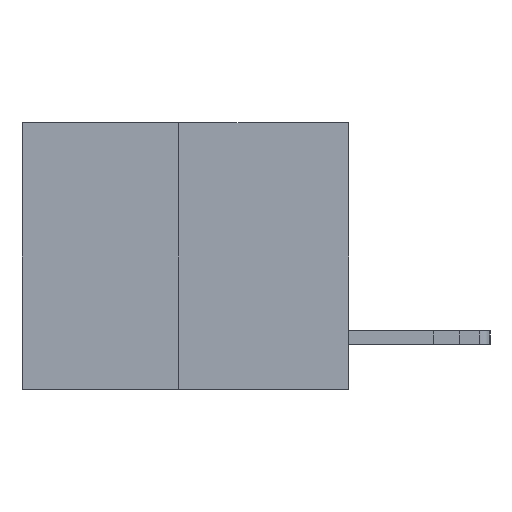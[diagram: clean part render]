
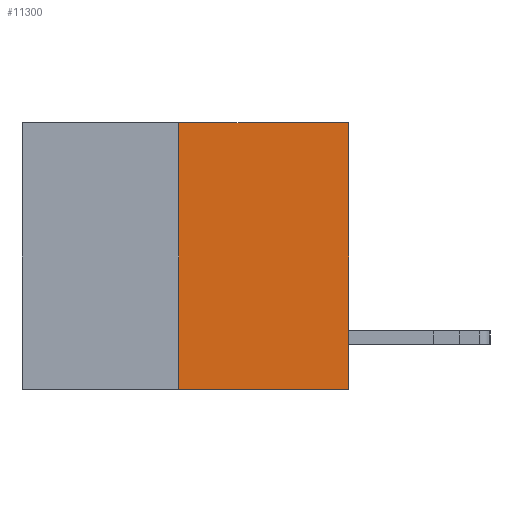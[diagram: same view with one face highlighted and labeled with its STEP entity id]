
A CAD part, left-side view. The second image highlights one B-rep face of the part: STEP entity #11300.
In plain terms, the highlighted planar face has unit normal (-1, 0, 0).
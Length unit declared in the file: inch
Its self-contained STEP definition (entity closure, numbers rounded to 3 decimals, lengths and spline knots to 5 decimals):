
#47 = ORIENTED_EDGE ( 'NONE', *, *, #2334, .F. ) ;
#474 = CARTESIAN_POINT ( 'NONE',  ( 0., 0., 0. ) ) ;
#1271 = VERTEX_POINT ( 'NONE', #4676 ) ;
#1705 = VECTOR ( 'NONE', #13946, 39.37008 ) ;
#1891 = EDGE_LOOP ( 'NONE', ( #47, #7938, #6065, #14692 ) ) ;
#2300 = FACE_OUTER_BOUND ( 'NONE', #1891, .T. ) ;
#2334 = EDGE_CURVE ( 'NONE', #10561, #4743, #7757, .T. ) ;
#2681 = EDGE_CURVE ( 'NONE', #1271, #6671, #13446, .T. ) ;
#3356 = CARTESIAN_POINT ( 'NONE',  ( 0., 0.6, 0. ) ) ;
#4238 = CARTESIAN_POINT ( 'NONE',  ( 0., 0.6, 0. ) ) ;
#4428 = EDGE_CURVE ( 'NONE', #10561, #1271, #6421, .T. ) ;
#4590 = CARTESIAN_POINT ( 'NONE',  ( 0., 0.312, -0.49 ) ) ;
#4676 = CARTESIAN_POINT ( 'NONE',  ( 0., 0., -0.49 ) ) ;
#4679 = AXIS2_PLACEMENT_3D ( 'NONE', #3356, #11577, #15067 ) ;
#4743 = VERTEX_POINT ( 'NONE', #8078 ) ;
#5913 = VECTOR ( 'NONE', #8720, 39.37008 ) ;
#6065 = ORIENTED_EDGE ( 'NONE', *, *, #2681, .T. ) ;
#6421 = LINE ( 'NONE', #14255, #8431 ) ;
#6671 = VERTEX_POINT ( 'NONE', #14829 ) ;
#7757 = LINE ( 'NONE', #4590, #1705 ) ;
#7938 = ORIENTED_EDGE ( 'NONE', *, *, #4428, .T. ) ;
#8078 = CARTESIAN_POINT ( 'NONE',  ( 0., 0.312, 0. ) ) ;
#8186 = CARTESIAN_POINT ( 'NONE',  ( 0., 0.312, -0.49 ) ) ;
#8431 = VECTOR ( 'NONE', #10799, 39.37008 ) ;
#8720 = DIRECTION ( 'NONE',  ( 0., 0., 1. ) ) ;
#9144 = PLANE ( 'NONE',  #4679 ) ;
#10342 = LINE ( 'NONE', #4238, #11990 ) ;
#10561 = VERTEX_POINT ( 'NONE', #8186 ) ;
#10799 = DIRECTION ( 'NONE',  ( 0., -1., 0. ) ) ;
#11300 = ADVANCED_FACE ( 'NONE', ( #2300 ), #9144, .F. ) ;
#11498 = DIRECTION ( 'NONE',  ( 0., -1., 0. ) ) ;
#11577 = DIRECTION ( 'NONE',  ( 1., 0., 0. ) ) ;
#11990 = VECTOR ( 'NONE', #11498, 39.37008 ) ;
#12763 = EDGE_CURVE ( 'NONE', #4743, #6671, #10342, .T. ) ;
#13446 = LINE ( 'NONE', #474, #5913 ) ;
#13946 = DIRECTION ( 'NONE',  ( 0., 0., 1. ) ) ;
#14255 = CARTESIAN_POINT ( 'NONE',  ( 0., 0.6, -0.49 ) ) ;
#14692 = ORIENTED_EDGE ( 'NONE', *, *, #12763, .F. ) ;
#14829 = CARTESIAN_POINT ( 'NONE',  ( 0., 0., 0. ) ) ;
#15067 = DIRECTION ( 'NONE',  ( 0., 0., -1. ) ) ;
